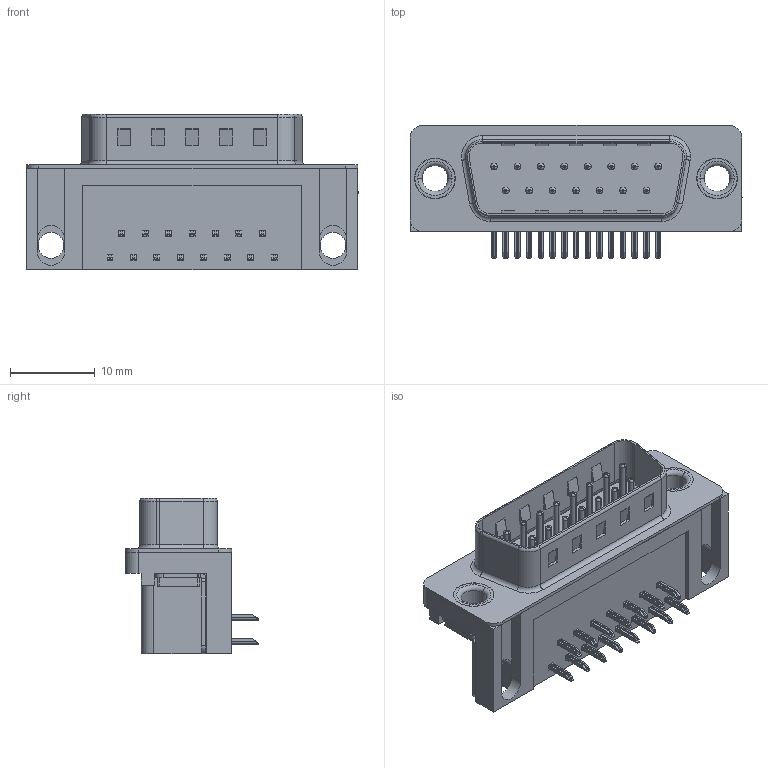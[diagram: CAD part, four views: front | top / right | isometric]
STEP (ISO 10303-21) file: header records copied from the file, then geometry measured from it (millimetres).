
FILE_DESCRIPTION (( 'STEP AP203' ), '1' );
FILE_NAME ('621-015-260-511.STEP', '2019-11-18T22:42:35', ( '' ), ( '' ), 'SwSTEP 2.0', 'SolidWorks 2016', '' );
FILE_SCHEMA (( 'CONFIG_CONTROL_DESIGN' ));
Length unit declared in the file: millimetre
Products named in the file (7): 621 Thru Hole Rivet; 621 Thru Hole Board Mount; 621 Housing_15 Socket; 621 Shell_15 Socket; 621-015-260-511; 621 Contact Bottom; 621 Contact Top
Assembly tree (21 placements, depth 2):
  621-015-260-511
    621 Housing_15 Socket
    621 Shell_15 Socket
    621 Contact Bottom  x7
    621 Contact Top  x8
    621 Thru Hole Board Mount  x2
    621 Thru Hole Rivet  x2
Bounding box: 39.22 x 15.73 x 18.4 mm (x, y, z)
Volume: 4400.7 mm3; surface area: 5613.7 mm2
Topology: 21 solids, 21 shells, 1435 faces, 3561 edges, 2205 vertices
Faces by surface type: plane 891, cylinder 427, torus 117
Entity records: 16601 total; most frequent: DIRECTION 2742, CARTESIAN_POINT 2684, ORIENTED_EDGE 2586, EDGE_CURVE 1293, AXIS2_PLACEMENT_3D 919, VECTOR 904, LINE 904, VERTEX_POINT 825
